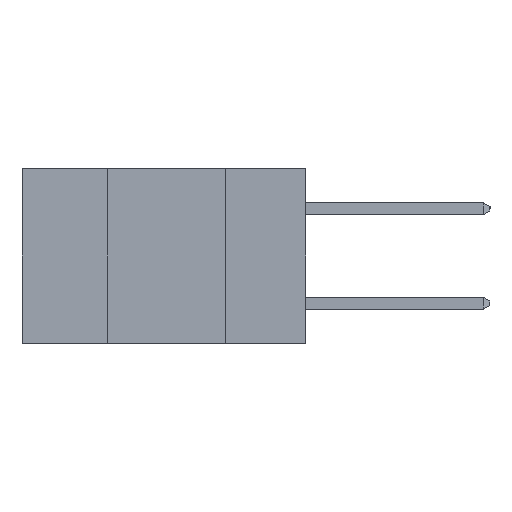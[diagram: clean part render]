
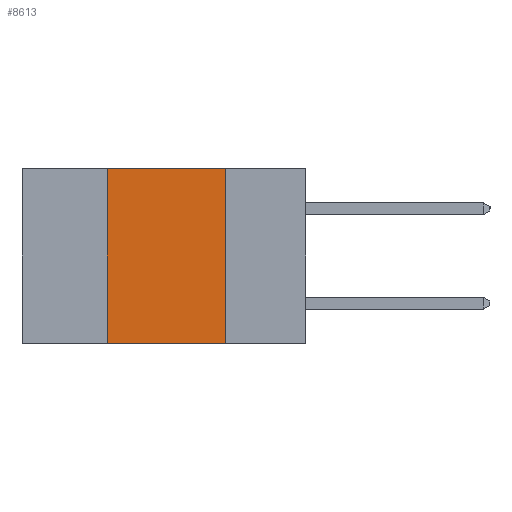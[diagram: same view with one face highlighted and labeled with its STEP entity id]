
A CAD part, left-side view. The second image highlights one B-rep face of the part: STEP entity #8613.
In plain terms, the highlighted planar face has unit normal (-1, 0, 0).
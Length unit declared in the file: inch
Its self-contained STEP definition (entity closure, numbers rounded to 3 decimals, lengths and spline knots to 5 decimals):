
#350 = CARTESIAN_POINT ( 'NONE',  ( 0., 0.42, -0.37 ) ) ;
#869 = CARTESIAN_POINT ( 'NONE',  ( 0., 0.17, 0. ) ) ;
#1731 = PLANE ( 'NONE',  #10896 ) ;
#1861 = DIRECTION ( 'NONE',  ( 0., 0., -1. ) ) ;
#2220 = LINE ( 'NONE', #350, #2521 ) ;
#2521 = VECTOR ( 'NONE', #3218, 39.37008 ) ;
#3075 = EDGE_CURVE ( 'NONE', #6666, #7654, #5207, .T. ) ;
#3218 = DIRECTION ( 'NONE',  ( 0., 0., 1. ) ) ;
#3881 = ORIENTED_EDGE ( 'NONE', *, *, #7088, .F. ) ;
#4964 = CARTESIAN_POINT ( 'NONE',  ( 0., 0.6, 0. ) ) ;
#4992 = CARTESIAN_POINT ( 'NONE',  ( 0., 0.42, -0.37 ) ) ;
#5207 = LINE ( 'NONE', #6197, #10881 ) ;
#5523 = CARTESIAN_POINT ( 'NONE',  ( 0., 0.6, 0. ) ) ;
#5641 = VERTEX_POINT ( 'NONE', #869 ) ;
#6036 = CARTESIAN_POINT ( 'NONE',  ( 0., 0.42, 0. ) ) ;
#6197 = CARTESIAN_POINT ( 'NONE',  ( 0., 0.6, -0.37 ) ) ;
#6414 = ORIENTED_EDGE ( 'NONE', *, *, #7190, .F. ) ;
#6648 = VERTEX_POINT ( 'NONE', #6036 ) ;
#6666 = VERTEX_POINT ( 'NONE', #4992 ) ;
#6941 = DIRECTION ( 'NONE',  ( 0., -1., 0. ) ) ;
#7088 = EDGE_CURVE ( 'NONE', #6666, #6648, #2220, .T. ) ;
#7190 = EDGE_CURVE ( 'NONE', #5641, #7654, #10733, .T. ) ;
#7654 = VERTEX_POINT ( 'NONE', #11022 ) ;
#8613 = ADVANCED_FACE ( 'NONE', ( #11412 ), #1731, .F. ) ;
#9365 = ORIENTED_EDGE ( 'NONE', *, *, #3075, .T. ) ;
#9765 = EDGE_CURVE ( 'NONE', #6648, #5641, #11721, .T. ) ;
#10733 = LINE ( 'NONE', #11035, #11460 ) ;
#10777 = EDGE_LOOP ( 'NONE', ( #6414, #10803, #3881, #9365 ) ) ;
#10803 = ORIENTED_EDGE ( 'NONE', *, *, #9765, .F. ) ;
#10881 = VECTOR ( 'NONE', #11971, 39.37008 ) ;
#10896 = AXIS2_PLACEMENT_3D ( 'NONE', #5523, #12174, #1861 ) ;
#11022 = CARTESIAN_POINT ( 'NONE',  ( 0., 0.17, -0.37 ) ) ;
#11035 = CARTESIAN_POINT ( 'NONE',  ( 0., 0.17, -0.37 ) ) ;
#11412 = FACE_OUTER_BOUND ( 'NONE', #10777, .T. ) ;
#11460 = VECTOR ( 'NONE', #11974, 39.37008 ) ;
#11497 = VECTOR ( 'NONE', #6941, 39.37008 ) ;
#11721 = LINE ( 'NONE', #4964, #11497 ) ;
#11971 = DIRECTION ( 'NONE',  ( 0., -1., 0. ) ) ;
#11974 = DIRECTION ( 'NONE',  ( 0., 0., -1. ) ) ;
#12174 = DIRECTION ( 'NONE',  ( 1., 0., 0. ) ) ;
